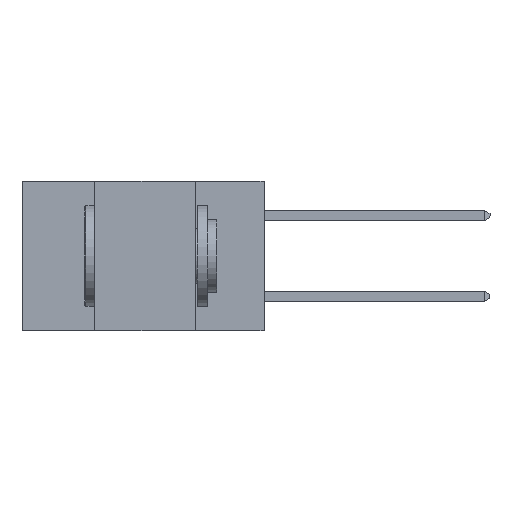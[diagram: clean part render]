
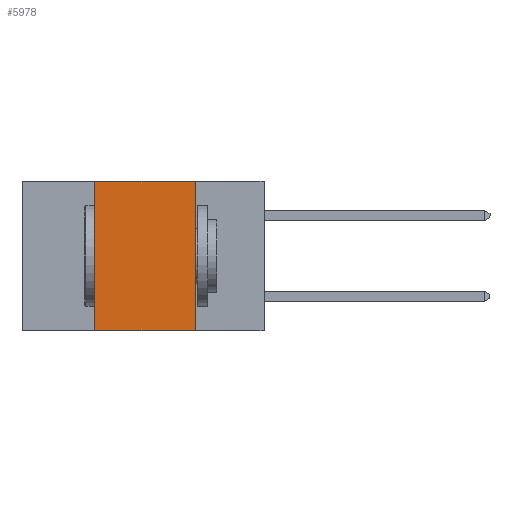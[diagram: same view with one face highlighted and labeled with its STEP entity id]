
A CAD part, left-side view. The second image highlights one B-rep face of the part: STEP entity #5978.
In plain terms, the highlighted planar face has unit normal (-1, 0, 0).
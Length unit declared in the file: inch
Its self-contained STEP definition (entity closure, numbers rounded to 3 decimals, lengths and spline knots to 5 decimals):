
#200 = VERTEX_POINT ( 'NONE', #2622 ) ;
#470 = VERTEX_POINT ( 'NONE', #22737 ) ;
#832 = EDGE_CURVE ( 'NONE', #8313, #200, #11462, .T. ) ;
#931 = CARTESIAN_POINT ( 'NONE',  ( 0., 0.6, 0. ) ) ;
#1181 = VECTOR ( 'NONE', #14033, 39.37008 ) ;
#2017 = LINE ( 'NONE', #931, #20352 ) ;
#2380 = EDGE_CURVE ( 'NONE', #470, #19030, #14897, .T. ) ;
#2622 = CARTESIAN_POINT ( 'NONE',  ( 0., 0.42, 0. ) ) ;
#5978 = ADVANCED_FACE ( 'NONE', ( #13384 ), #19773, .F. ) ;
#7116 = CARTESIAN_POINT ( 'NONE',  ( 0., 0.17, -0.37 ) ) ;
#7386 = DIRECTION ( 'NONE',  ( 0., 0., -1. ) ) ;
#7457 = DIRECTION ( 'NONE',  ( 1., 0., 0. ) ) ;
#7854 = CARTESIAN_POINT ( 'NONE',  ( 0., 0.6, 0. ) ) ;
#7866 = VECTOR ( 'NONE', #21481, 39.37008 ) ;
#8125 = ORIENTED_EDGE ( 'NONE', *, *, #8713, .T. ) ;
#8313 = VERTEX_POINT ( 'NONE', #13502 ) ;
#8713 = EDGE_CURVE ( 'NONE', #8313, #19030, #17264, .T. ) ;
#11462 = LINE ( 'NONE', #21081, #20812 ) ;
#11707 = ORIENTED_EDGE ( 'NONE', *, *, #832, .F. ) ;
#12715 = CARTESIAN_POINT ( 'NONE',  ( 0., 0.6, -0.37 ) ) ;
#13384 = FACE_OUTER_BOUND ( 'NONE', #17755, .T. ) ;
#13502 = CARTESIAN_POINT ( 'NONE',  ( 0., 0.42, -0.37 ) ) ;
#14033 = DIRECTION ( 'NONE',  ( 0., 0., -1. ) ) ;
#14403 = AXIS2_PLACEMENT_3D ( 'NONE', #7854, #7457, #7386 ) ;
#14405 = DIRECTION ( 'NONE',  ( 0., 0., 1. ) ) ;
#14897 = LINE ( 'NONE', #15426, #1181 ) ;
#15291 = ORIENTED_EDGE ( 'NONE', *, *, #21502, .F. ) ;
#15426 = CARTESIAN_POINT ( 'NONE',  ( 0., 0.17, 0. ) ) ;
#17264 = LINE ( 'NONE', #12715, #7866 ) ;
#17755 = EDGE_LOOP ( 'NONE', ( #18867, #15291, #11707, #8125 ) ) ;
#18867 = ORIENTED_EDGE ( 'NONE', *, *, #2380, .F. ) ;
#19030 = VERTEX_POINT ( 'NONE', #7116 ) ;
#19773 = PLANE ( 'NONE',  #14403 ) ;
#20352 = VECTOR ( 'NONE', #20628, 39.37008 ) ;
#20628 = DIRECTION ( 'NONE',  ( 0., -1., 0. ) ) ;
#20812 = VECTOR ( 'NONE', #14405, 39.37008 ) ;
#21081 = CARTESIAN_POINT ( 'NONE',  ( 0., 0.42, 0. ) ) ;
#21481 = DIRECTION ( 'NONE',  ( 0., -1., 0. ) ) ;
#21502 = EDGE_CURVE ( 'NONE', #200, #470, #2017, .T. ) ;
#22737 = CARTESIAN_POINT ( 'NONE',  ( 0., 0.17, 0. ) ) ;
